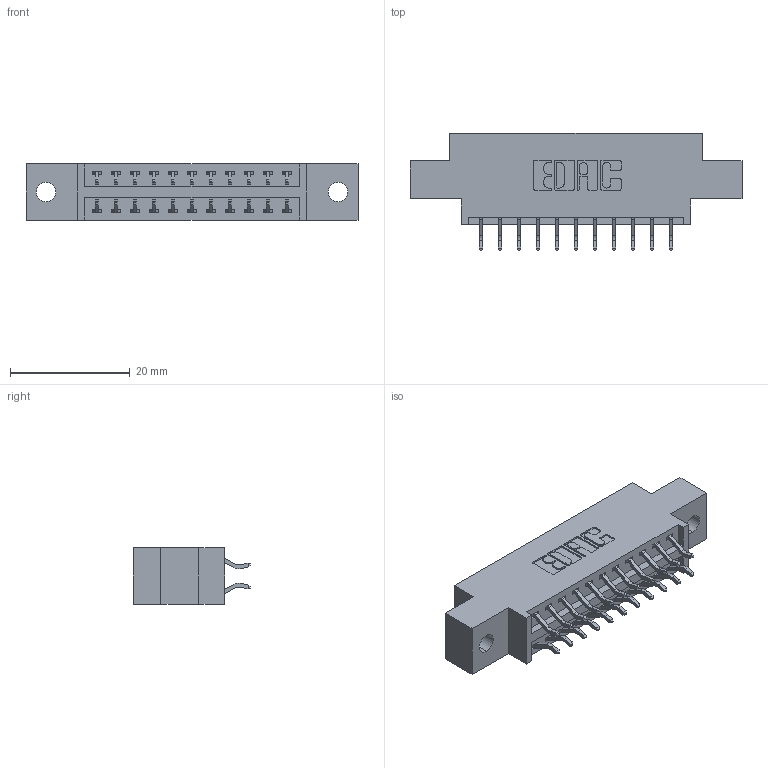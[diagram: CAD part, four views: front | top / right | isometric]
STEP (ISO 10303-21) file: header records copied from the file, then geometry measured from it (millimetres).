
FILE_DESCRIPTION (( 'STEP AP203' ), '1' );
FILE_NAME ('396-022-556-802.STEP', '2018-09-01T10:23:34', ( '' ), ( '' ), 'SwSTEP 2.0', 'SolidWorks 2016', '' );
FILE_SCHEMA (( 'CONFIG_CONTROL_DESIGN' ));
Length unit declared in the file: inch
Products named in the file (3): 345-292-001_556 Tail; 396-022-556-802; 346 Part_0.170 Offset - 0.128 Dia
Assembly tree (23 placements, depth 2):
  396-022-556-802
    346 Part_0.170 Offset - 0.128 Dia
    345-292-001_556 Tail  x22
Bounding box: 55.5 x 19.57 x 9.4 mm (x, y, z)
Volume: 4978.9 mm3; surface area: 6246.5 mm2
Topology: 23 solids, 23 shells, 1402 faces, 4147 edges, 2734 vertices
Faces by surface type: plane 938, cylinder 464
Entity records: 11707 total; most frequent: CARTESIAN_POINT 1988, ORIENTED_EDGE 1910, DIRECTION 1791, EDGE_CURVE 955, LINE 771, VECTOR 771, VERTEX_POINT 634, AXIS2_PLACEMENT_3D 510
